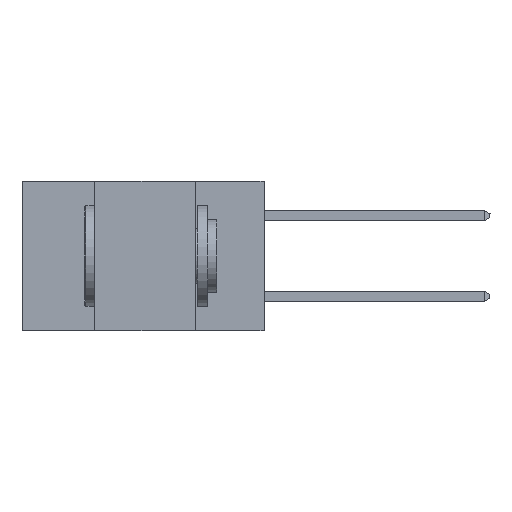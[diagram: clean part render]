
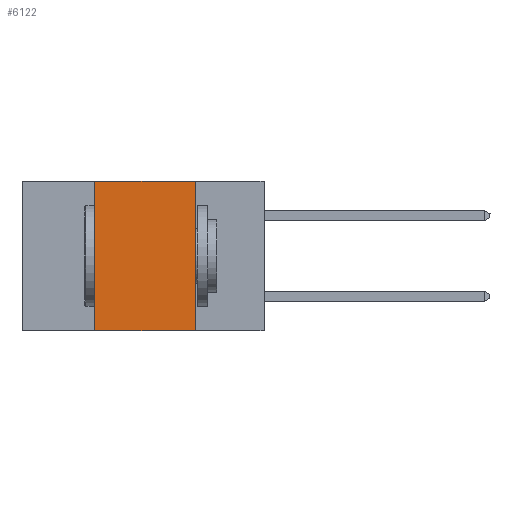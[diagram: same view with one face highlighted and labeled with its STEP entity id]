
A CAD part, left-side view. The second image highlights one B-rep face of the part: STEP entity #6122.
In plain terms, the highlighted planar face has unit normal (-1, 0, 0).
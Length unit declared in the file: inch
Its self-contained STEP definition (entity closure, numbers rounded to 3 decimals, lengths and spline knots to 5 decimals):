
#952 = CARTESIAN_POINT ( 'NONE',  ( 0., 0.6, 0. ) ) ;
#1028 = AXIS2_PLACEMENT_3D ( 'NONE', #6529, #1666, #19480 ) ;
#1180 = LINE ( 'NONE', #952, #20536 ) ;
#1666 = DIRECTION ( 'NONE',  ( 1., 0., 0. ) ) ;
#2793 = CARTESIAN_POINT ( 'NONE',  ( 0., 0.42, 0. ) ) ;
#3000 = CARTESIAN_POINT ( 'NONE',  ( 0., 0.42, -0.37 ) ) ;
#4167 = DIRECTION ( 'NONE',  ( 0., -1., 0. ) ) ;
#4507 = ORIENTED_EDGE ( 'NONE', *, *, #11799, .F. ) ;
#5149 = DIRECTION ( 'NONE',  ( 0., 0., 1. ) ) ;
#6122 = ADVANCED_FACE ( 'NONE', ( #11875 ), #9990, .F. ) ;
#6363 = LINE ( 'NONE', #16755, #11986 ) ;
#6529 = CARTESIAN_POINT ( 'NONE',  ( 0., 0.6, 0. ) ) ;
#7783 = EDGE_CURVE ( 'NONE', #20839, #12613, #14110, .T. ) ;
#7997 = EDGE_CURVE ( 'NONE', #13122, #12613, #20680, .T. ) ;
#8502 = VECTOR ( 'NONE', #12991, 39.37008 ) ;
#9275 = VECTOR ( 'NONE', #15667, 39.37008 ) ;
#9345 = CARTESIAN_POINT ( 'NONE',  ( 0., 0.17, -0.37 ) ) ;
#9990 = PLANE ( 'NONE',  #1028 ) ;
#11198 = ORIENTED_EDGE ( 'NONE', *, *, #7997, .F. ) ;
#11628 = ORIENTED_EDGE ( 'NONE', *, *, #7783, .T. ) ;
#11640 = CARTESIAN_POINT ( 'NONE',  ( 0., 0.17, 0. ) ) ;
#11799 = EDGE_CURVE ( 'NONE', #20804, #13122, #1180, .T. ) ;
#11875 = FACE_OUTER_BOUND ( 'NONE', #12632, .T. ) ;
#11986 = VECTOR ( 'NONE', #5149, 39.37008 ) ;
#12613 = VERTEX_POINT ( 'NONE', #9345 ) ;
#12632 = EDGE_LOOP ( 'NONE', ( #11198, #4507, #13783, #11628 ) ) ;
#12991 = DIRECTION ( 'NONE',  ( 0., 0., -1. ) ) ;
#13122 = VERTEX_POINT ( 'NONE', #20388 ) ;
#13783 = ORIENTED_EDGE ( 'NONE', *, *, #15945, .F. ) ;
#14110 = LINE ( 'NONE', #18780, #9275 ) ;
#15667 = DIRECTION ( 'NONE',  ( 0., -1., 0. ) ) ;
#15945 = EDGE_CURVE ( 'NONE', #20839, #20804, #6363, .T. ) ;
#16755 = CARTESIAN_POINT ( 'NONE',  ( 0., 0.42, 0. ) ) ;
#18780 = CARTESIAN_POINT ( 'NONE',  ( 0., 0.6, -0.37 ) ) ;
#19480 = DIRECTION ( 'NONE',  ( 0., 0., -1. ) ) ;
#20388 = CARTESIAN_POINT ( 'NONE',  ( 0., 0.17, 0. ) ) ;
#20536 = VECTOR ( 'NONE', #4167, 39.37008 ) ;
#20680 = LINE ( 'NONE', #11640, #8502 ) ;
#20804 = VERTEX_POINT ( 'NONE', #2793 ) ;
#20839 = VERTEX_POINT ( 'NONE', #3000 ) ;
